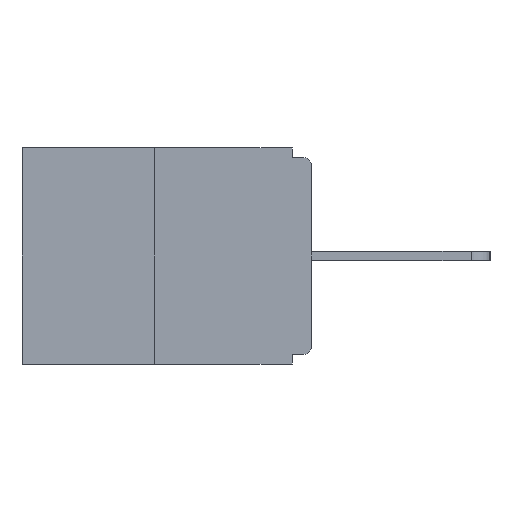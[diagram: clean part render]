
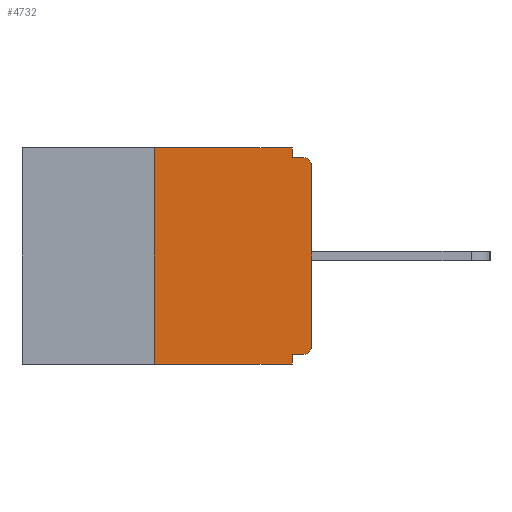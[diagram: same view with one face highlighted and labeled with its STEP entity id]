
A CAD part, left-side view. The second image highlights one B-rep face of the part: STEP entity #4732.
In plain terms, the highlighted planar face has unit normal (-1, 0, 0).
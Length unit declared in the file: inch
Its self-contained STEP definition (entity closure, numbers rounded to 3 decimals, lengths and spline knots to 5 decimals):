
#27 = CARTESIAN_POINT ( 'NONE',  ( 0., 0.031, -0.343 ) ) ;
#785 = EDGE_CURVE ( 'NONE', #16714, #1918, #7127, .T. ) ;
#885 = ORIENTED_EDGE ( 'NONE', *, *, #16651, .T. ) ;
#924 = DIRECTION ( 'NONE',  ( 0., 0., -1. ) ) ;
#940 = DIRECTION ( 'NONE',  ( 0., 1., 0. ) ) ;
#1201 = CARTESIAN_POINT ( 'NONE',  ( 0., 0.25, 0. ) ) ;
#1918 = VERTEX_POINT ( 'NONE', #14251 ) ;
#2203 = DIRECTION ( 'NONE',  ( 0., 0., -1. ) ) ;
#2569 = VERTEX_POINT ( 'NONE', #7671 ) ;
#2734 = CARTESIAN_POINT ( 'NONE',  ( 0., 0., 0. ) ) ;
#3439 = DIRECTION ( 'NONE',  ( 0., -1., 0. ) ) ;
#3681 = DIRECTION ( 'NONE',  ( 0., -1., 0. ) ) ;
#3718 = ORIENTED_EDGE ( 'NONE', *, *, #17886, .T. ) ;
#3957 = VECTOR ( 'NONE', #940, 39.37008 ) ;
#4148 = ORIENTED_EDGE ( 'NONE', *, *, #18204, .F. ) ;
#4446 = CARTESIAN_POINT ( 'NONE',  ( 0., 0.031, -0.015 ) ) ;
#4732 = ADVANCED_FACE ( 'NONE', ( #18348 ), #20406, .F. ) ;
#4821 = EDGE_CURVE ( 'NONE', #25144, #16714, #13132, .T. ) ;
#5705 = VERTEX_POINT ( 'NONE', #19605 ) ;
#6934 = DIRECTION ( 'NONE',  ( -1., 0., 0. ) ) ;
#7127 = LINE ( 'NONE', #15432, #19381 ) ;
#7295 = VECTOR ( 'NONE', #12798, 39.37008 ) ;
#7410 = AXIS2_PLACEMENT_3D ( 'NONE', #14346, #22140, #924 ) ;
#7499 = VERTEX_POINT ( 'NONE', #23261 ) ;
#7671 = CARTESIAN_POINT ( 'NONE',  ( 0., 0.015, -0.015 ) ) ;
#9322 = LINE ( 'NONE', #9440, #18564 ) ;
#9440 = CARTESIAN_POINT ( 'NONE',  ( 0., 0.46, -0.343 ) ) ;
#9901 = EDGE_CURVE ( 'NONE', #1918, #11601, #18940, .T. ) ;
#10135 = CARTESIAN_POINT ( 'NONE',  ( 0., 0.031, -0.328 ) ) ;
#10145 = LINE ( 'NONE', #12200, #3957 ) ;
#11034 = ORIENTED_EDGE ( 'NONE', *, *, #9901, .F. ) ;
#11077 = CARTESIAN_POINT ( 'NONE',  ( 0., 0.25, 0. ) ) ;
#11601 = VERTEX_POINT ( 'NONE', #4446 ) ;
#12176 = AXIS2_PLACEMENT_3D ( 'NONE', #24468, #6934, #20611 ) ;
#12200 = CARTESIAN_POINT ( 'NONE',  ( 0., 0., -0.328 ) ) ;
#12333 = ORIENTED_EDGE ( 'NONE', *, *, #4821, .F. ) ;
#12462 = LINE ( 'NONE', #2734, #23154 ) ;
#12509 = EDGE_CURVE ( 'NONE', #25144, #19156, #9322, .T. ) ;
#12798 = DIRECTION ( 'NONE',  ( 0., -1., 0. ) ) ;
#12970 = ORIENTED_EDGE ( 'NONE', *, *, #785, .F. ) ;
#13033 = AXIS2_PLACEMENT_3D ( 'NONE', #24519, #14653, #16679 ) ;
#13132 = LINE ( 'NONE', #11077, #20405 ) ;
#13269 = EDGE_CURVE ( 'NONE', #21873, #19156, #17526, .T. ) ;
#13305 = ORIENTED_EDGE ( 'NONE', *, *, #12509, .T. ) ;
#13387 = DIRECTION ( 'NONE',  ( 0., 0., 1. ) ) ;
#13431 = EDGE_CURVE ( 'NONE', #5705, #7499, #14755, .T. ) ;
#14047 = ORIENTED_EDGE ( 'NONE', *, *, #13431, .T. ) ;
#14251 = CARTESIAN_POINT ( 'NONE',  ( 0., 0.031, 0. ) ) ;
#14346 = CARTESIAN_POINT ( 'NONE',  ( 0., 0.015, -0.313 ) ) ;
#14653 = DIRECTION ( 'NONE',  ( 1., 0., 0. ) ) ;
#14755 = CIRCLE ( 'NONE', #7410, 0.015 ) ;
#14847 = CARTESIAN_POINT ( 'NONE',  ( 0., 0.031, 0. ) ) ;
#14980 = DIRECTION ( 'NONE',  ( 0., 0., -1. ) ) ;
#15303 = EDGE_CURVE ( 'NONE', #5705, #21873, #10145, .T. ) ;
#15432 = CARTESIAN_POINT ( 'NONE',  ( 0., 0.46, 0. ) ) ;
#15868 = CARTESIAN_POINT ( 'NONE',  ( 0., 0.25, -0.343 ) ) ;
#16651 = EDGE_CURVE ( 'NONE', #7499, #19923, #12462, .T. ) ;
#16679 = DIRECTION ( 'NONE',  ( 0., 0., -1. ) ) ;
#16714 = VERTEX_POINT ( 'NONE', #1201 ) ;
#17173 = ORIENTED_EDGE ( 'NONE', *, *, #15303, .F. ) ;
#17526 = LINE ( 'NONE', #27, #18417 ) ;
#17688 = EDGE_LOOP ( 'NONE', ( #12970, #12333, #13305, #20210, #17173, #14047, #885, #3718, #4148, #11034 ) ) ;
#17886 = EDGE_CURVE ( 'NONE', #19923, #2569, #23209, .T. ) ;
#18204 = EDGE_CURVE ( 'NONE', #11601, #2569, #23670, .T. ) ;
#18348 = FACE_OUTER_BOUND ( 'NONE', #17688, .T. ) ;
#18417 = VECTOR ( 'NONE', #2203, 39.37008 ) ;
#18564 = VECTOR ( 'NONE', #3439, 39.37008 ) ;
#18940 = LINE ( 'NONE', #14847, #24204 ) ;
#19156 = VERTEX_POINT ( 'NONE', #23822 ) ;
#19381 = VECTOR ( 'NONE', #3681, 39.37008 ) ;
#19605 = CARTESIAN_POINT ( 'NONE',  ( 0., 0.015, -0.328 ) ) ;
#19923 = VERTEX_POINT ( 'NONE', #24012 ) ;
#20210 = ORIENTED_EDGE ( 'NONE', *, *, #13269, .F. ) ;
#20364 = DIRECTION ( 'NONE',  ( 0., 0., 1. ) ) ;
#20405 = VECTOR ( 'NONE', #13387, 39.37008 ) ;
#20406 = PLANE ( 'NONE',  #13033 ) ;
#20611 = DIRECTION ( 'NONE',  ( 0., 0., -1. ) ) ;
#21873 = VERTEX_POINT ( 'NONE', #10135 ) ;
#22140 = DIRECTION ( 'NONE',  ( -1., 0., 0. ) ) ;
#23154 = VECTOR ( 'NONE', #20364, 39.37008 ) ;
#23209 = CIRCLE ( 'NONE', #12176, 0.015 ) ;
#23261 = CARTESIAN_POINT ( 'NONE',  ( 0., 0., -0.313 ) ) ;
#23670 = LINE ( 'NONE', #24436, #7295 ) ;
#23822 = CARTESIAN_POINT ( 'NONE',  ( 0., 0.031, -0.343 ) ) ;
#24012 = CARTESIAN_POINT ( 'NONE',  ( 0., 0., -0.03 ) ) ;
#24204 = VECTOR ( 'NONE', #14980, 39.37008 ) ;
#24436 = CARTESIAN_POINT ( 'NONE',  ( 0., 0., -0.015 ) ) ;
#24468 = CARTESIAN_POINT ( 'NONE',  ( 0., 0.015, -0.03 ) ) ;
#24519 = CARTESIAN_POINT ( 'NONE',  ( 0., 0.46, 0. ) ) ;
#25144 = VERTEX_POINT ( 'NONE', #15868 ) ;
